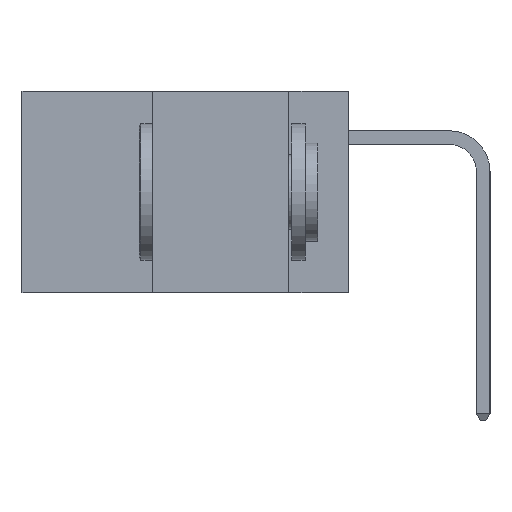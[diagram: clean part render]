
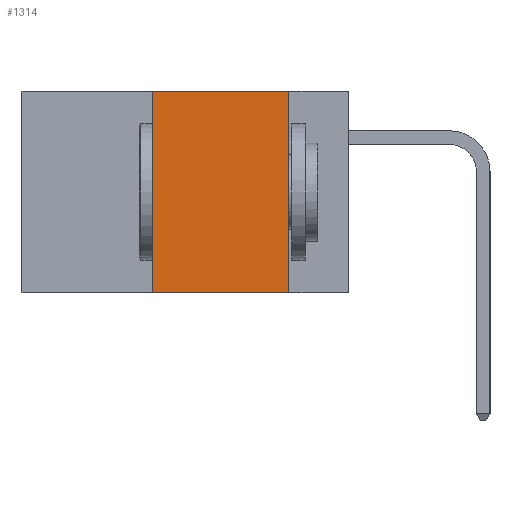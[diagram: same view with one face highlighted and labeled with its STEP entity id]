
A CAD part, left-side view. The second image highlights one B-rep face of the part: STEP entity #1314.
In plain terms, the highlighted planar face has unit normal (-1, 0, 0).
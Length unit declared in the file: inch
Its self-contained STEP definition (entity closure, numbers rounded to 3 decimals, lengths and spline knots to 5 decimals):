
#7 = CARTESIAN_POINT ( 'NONE',  ( 0., 0.6, 0. ) ) ;
#206 = CARTESIAN_POINT ( 'NONE',  ( 0., 0.6, -0.37 ) ) ;
#1314 = ADVANCED_FACE ( 'NONE', ( #4234 ), #6019, .F. ) ;
#1336 = EDGE_CURVE ( 'NONE', #9987, #7321, #7832, .T. ) ;
#1664 = VECTOR ( 'NONE', #4648, 39.37008 ) ;
#2180 = EDGE_CURVE ( 'NONE', #7321, #4763, #2233, .T. ) ;
#2233 = LINE ( 'NONE', #8781, #8270 ) ;
#2887 = AXIS2_PLACEMENT_3D ( 'NONE', #7, #4316, #6385 ) ;
#3374 = CARTESIAN_POINT ( 'NONE',  ( 0., 0.36, 0. ) ) ;
#3476 = CARTESIAN_POINT ( 'NONE',  ( 0., 0.11, 0. ) ) ;
#3666 = VECTOR ( 'NONE', #4662, 39.37008 ) ;
#4234 = FACE_OUTER_BOUND ( 'NONE', #7040, .T. ) ;
#4316 = DIRECTION ( 'NONE',  ( 1., 0., 0. ) ) ;
#4648 = DIRECTION ( 'NONE',  ( 0., 0., 1. ) ) ;
#4662 = DIRECTION ( 'NONE',  ( 0., -1., 0. ) ) ;
#4763 = VERTEX_POINT ( 'NONE', #9698 ) ;
#5186 = ORIENTED_EDGE ( 'NONE', *, *, #9688, .F. ) ;
#5251 = ORIENTED_EDGE ( 'NONE', *, *, #2180, .F. ) ;
#5505 = ORIENTED_EDGE ( 'NONE', *, *, #1336, .F. ) ;
#5536 = ORIENTED_EDGE ( 'NONE', *, *, #5541, .T. ) ;
#5541 = EDGE_CURVE ( 'NONE', #9987, #8805, #9396, .T. ) ;
#6019 = PLANE ( 'NONE',  #2887 ) ;
#6385 = DIRECTION ( 'NONE',  ( 0., 0., -1. ) ) ;
#7040 = EDGE_LOOP ( 'NONE', ( #5186, #5251, #5505, #5536 ) ) ;
#7321 = VERTEX_POINT ( 'NONE', #9701 ) ;
#7832 = LINE ( 'NONE', #3374, #1664 ) ;
#7914 = VECTOR ( 'NONE', #8824, 39.37008 ) ;
#8147 = LINE ( 'NONE', #3476, #7914 ) ;
#8270 = VECTOR ( 'NONE', #8981, 39.37008 ) ;
#8781 = CARTESIAN_POINT ( 'NONE',  ( 0., 0.6, 0. ) ) ;
#8805 = VERTEX_POINT ( 'NONE', #9087 ) ;
#8824 = DIRECTION ( 'NONE',  ( 0., 0., -1. ) ) ;
#8981 = DIRECTION ( 'NONE',  ( 0., -1., 0. ) ) ;
#9087 = CARTESIAN_POINT ( 'NONE',  ( 0., 0.11, -0.37 ) ) ;
#9396 = LINE ( 'NONE', #206, #3666 ) ;
#9688 = EDGE_CURVE ( 'NONE', #4763, #8805, #8147, .T. ) ;
#9698 = CARTESIAN_POINT ( 'NONE',  ( 0., 0.11, 0. ) ) ;
#9701 = CARTESIAN_POINT ( 'NONE',  ( 0., 0.36, 0. ) ) ;
#9776 = CARTESIAN_POINT ( 'NONE',  ( 0., 0.36, -0.37 ) ) ;
#9987 = VERTEX_POINT ( 'NONE', #9776 ) ;
